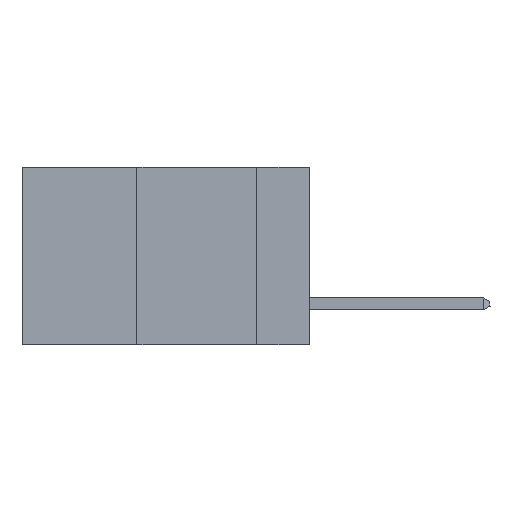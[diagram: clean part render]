
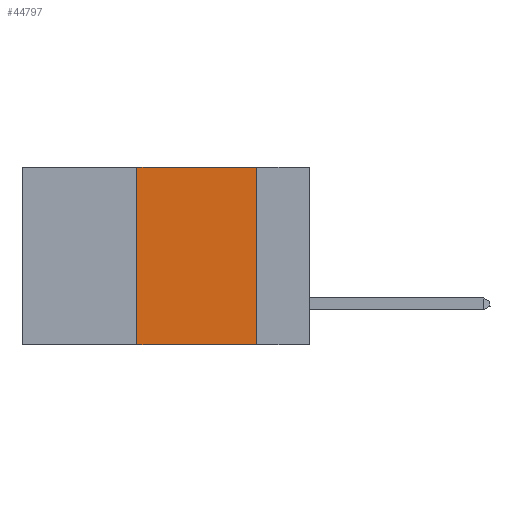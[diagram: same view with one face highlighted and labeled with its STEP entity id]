
A CAD part, left-side view. The second image highlights one B-rep face of the part: STEP entity #44797.
In plain terms, the highlighted planar face has unit normal (-1, 0, 0).
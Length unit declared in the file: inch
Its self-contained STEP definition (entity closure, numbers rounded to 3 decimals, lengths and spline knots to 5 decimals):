
#171 = EDGE_CURVE ( 'NONE', #39815, #49769, #43843, .T. ) ;
#2986 = AXIS2_PLACEMENT_3D ( 'NONE', #36837, #11087, #27209 ) ;
#3563 = DIRECTION ( 'NONE',  ( 0., 0., -1. ) ) ;
#7164 = PLANE ( 'NONE',  #2986 ) ;
#7655 = VECTOR ( 'NONE', #3563, 39.37008 ) ;
#8630 = EDGE_LOOP ( 'NONE', ( #22580, #33589, #47974, #49265 ) ) ;
#9755 = CARTESIAN_POINT ( 'NONE',  ( 0., 0.11, -0.37 ) ) ;
#9896 = VECTOR ( 'NONE', #35238, 39.37008 ) ;
#9897 = DIRECTION ( 'NONE',  ( 0., -1., 0. ) ) ;
#11087 = DIRECTION ( 'NONE',  ( 1., 0., 0. ) ) ;
#11318 = CARTESIAN_POINT ( 'NONE',  ( 0., 0.11, 0. ) ) ;
#13285 = CARTESIAN_POINT ( 'NONE',  ( 0., 0.11, 0. ) ) ;
#14227 = CARTESIAN_POINT ( 'NONE',  ( 0., 0.6, -0.37 ) ) ;
#15124 = VERTEX_POINT ( 'NONE', #48174 ) ;
#16410 = EDGE_CURVE ( 'NONE', #15124, #49769, #21870, .T. ) ;
#20874 = CARTESIAN_POINT ( 'NONE',  ( 0., 0.36, 0. ) ) ;
#21516 = VECTOR ( 'NONE', #36755, 39.37008 ) ;
#21870 = LINE ( 'NONE', #14227, #29937 ) ;
#22418 = FACE_OUTER_BOUND ( 'NONE', #8630, .T. ) ;
#22580 = ORIENTED_EDGE ( 'NONE', *, *, #171, .F. ) ;
#22861 = LINE ( 'NONE', #20874, #21516 ) ;
#27209 = DIRECTION ( 'NONE',  ( 0., 0., -1. ) ) ;
#29937 = VECTOR ( 'NONE', #9897, 39.37008 ) ;
#30811 = CARTESIAN_POINT ( 'NONE',  ( 0., 0.6, 0. ) ) ;
#32067 = EDGE_CURVE ( 'NONE', #15124, #47452, #22861, .T. ) ;
#33589 = ORIENTED_EDGE ( 'NONE', *, *, #50748, .F. ) ;
#35238 = DIRECTION ( 'NONE',  ( 0., -1., 0. ) ) ;
#36755 = DIRECTION ( 'NONE',  ( 0., 0., 1. ) ) ;
#36837 = CARTESIAN_POINT ( 'NONE',  ( 0., 0.6, 0. ) ) ;
#39815 = VERTEX_POINT ( 'NONE', #13285 ) ;
#40063 = LINE ( 'NONE', #30811, #9896 ) ;
#43843 = LINE ( 'NONE', #11318, #7655 ) ;
#44797 = ADVANCED_FACE ( 'NONE', ( #22418 ), #7164, .F. ) ;
#44935 = CARTESIAN_POINT ( 'NONE',  ( 0., 0.36, 0. ) ) ;
#47452 = VERTEX_POINT ( 'NONE', #44935 ) ;
#47974 = ORIENTED_EDGE ( 'NONE', *, *, #32067, .F. ) ;
#48174 = CARTESIAN_POINT ( 'NONE',  ( 0., 0.36, -0.37 ) ) ;
#49265 = ORIENTED_EDGE ( 'NONE', *, *, #16410, .T. ) ;
#49769 = VERTEX_POINT ( 'NONE', #9755 ) ;
#50748 = EDGE_CURVE ( 'NONE', #47452, #39815, #40063, .T. ) ;
